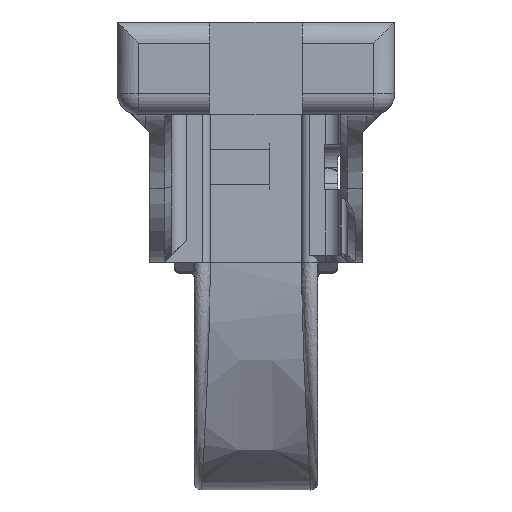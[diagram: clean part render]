
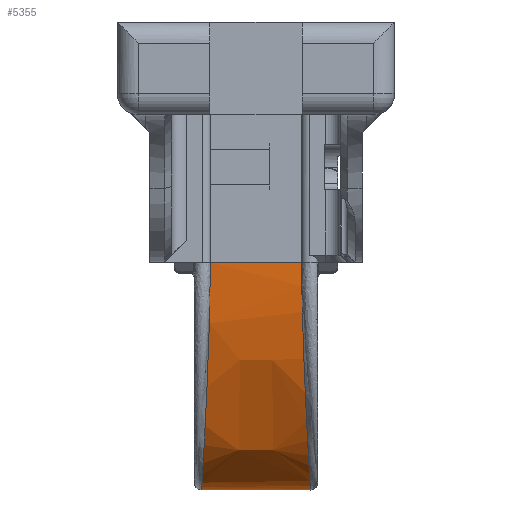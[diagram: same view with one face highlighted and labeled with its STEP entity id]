
A CAD part, left-side view. The second image highlights one B-rep face of the part: STEP entity #5355.
In plain terms, the highlighted free-form (B-spline) face has degree [3, 3] with [4, 4] control points.
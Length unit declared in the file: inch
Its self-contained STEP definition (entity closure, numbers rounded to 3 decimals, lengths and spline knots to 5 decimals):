
#70 = VERTEX_POINT ( 'NONE', #4380 ) ;
#248 = CARTESIAN_POINT ( 'NONE',  ( -0.38772, -0.25252, -3.07902 ) ) ;
#508 = CARTESIAN_POINT ( 'NONE',  ( -0.16815, -0.30113, -3.85823 ) ) ;
#726 = EDGE_CURVE ( 'NONE', #10322, #70, #4821, .T. ) ;
#775 = B_SPLINE_SURFACE_WITH_KNOTS ( 'NONE', 3, 3, ( 
 ( #8482, #3906, #8348, #7526 ),
 ( #4194, #6306, #5757, #4771 ),
 ( #4387, #3349, #3113, #1288 ),
 ( #785, #508, #248, #13104 ) ),
 .UNSPECIFIED., .F., .F., .F.,
 ( 4, 4 ),
 ( 4, 4 ),
 ( 0., 1. ),
 ( 0., 1. ),
 .UNSPECIFIED. ) ;
#785 = CARTESIAN_POINT ( 'NONE',  ( 0.31264, -0.30113, -3.85823 ) ) ;
#1165 = CARTESIAN_POINT ( 'NONE',  ( -0.38772, 0.25252, -2.59823 ) ) ;
#1271 = EDGE_LOOP ( 'NONE', ( #6556, #1324, #7472, #7667 ) ) ;
#1288 = CARTESIAN_POINT ( 'NONE',  ( -0.38772, -0.08417, -2.59823 ) ) ;
#1324 = ORIENTED_EDGE ( 'NONE', *, *, #9074, .T. ) ;
#1692 = B_SPLINE_CURVE_WITH_KNOTS ( 'NONE', 3,
 ( #6113, #6970, #6073, #6039 ),
 .UNSPECIFIED., .F., .F.,
 ( 4, 4 ),
 ( 0., 1. ),
 .UNSPECIFIED. ) ;
#1885 = CARTESIAN_POINT ( 'NONE',  ( 0.31264, 0.73097, -3.85823 ) ) ;
#2509 = CARTESIAN_POINT ( 'NONE',  ( -0.38772, -0.25252, -2.59823 ) ) ;
#2589 = DIRECTION ( 'NONE',  ( 0., 1., 0. ) ) ;
#2643 = CARTESIAN_POINT ( 'NONE',  ( -0.38772, 0., -2.59823 ) ) ;
#2877 = VERTEX_POINT ( 'NONE', #2509 ) ;
#3113 = CARTESIAN_POINT ( 'NONE',  ( -0.38772, -0.08417, -3.07902 ) ) ;
#3349 = CARTESIAN_POINT ( 'NONE',  ( -0.16815, -0.10038, -3.85823 ) ) ;
#3477 = CARTESIAN_POINT ( 'NONE',  ( -0.38772, 0.25252, -2.59823 ) ) ;
#3906 = CARTESIAN_POINT ( 'NONE',  ( -0.16815, 0.30113, -3.85823 ) ) ;
#4194 = CARTESIAN_POINT ( 'NONE',  ( 0.31264, 0.10038, -3.85823 ) ) ;
#4315 = CARTESIAN_POINT ( 'NONE',  ( 0.31264, 0.30113, -3.85823 ) ) ;
#4380 = CARTESIAN_POINT ( 'NONE',  ( 0.31264, -0.30113, -3.85823 ) ) ;
#4387 = CARTESIAN_POINT ( 'NONE',  ( 0.31264, -0.10038, -3.85823 ) ) ;
#4621 = VECTOR ( 'NONE', #12968, 39.37008 ) ;
#4771 = CARTESIAN_POINT ( 'NONE',  ( -0.38772, 0.08417, -2.59823 ) ) ;
#4796 = B_SPLINE_CURVE_WITH_KNOTS ( 'NONE', 3,
 ( #3477, #11599, #5252, #5219 ),
 .UNSPECIFIED., .F., .F.,
 ( 4, 4 ),
 ( 0., 1. ),
 .UNSPECIFIED. ) ;
#4821 = LINE ( 'NONE', #1885, #4621 ) ;
#5219 = CARTESIAN_POINT ( 'NONE',  ( 0.31264, 0.30113, -3.85823 ) ) ;
#5252 = CARTESIAN_POINT ( 'NONE',  ( -0.16815, 0.30113, -3.85823 ) ) ;
#5355 = ADVANCED_FACE ( 'NONE', ( #12349 ), #775, .T. ) ;
#5757 = CARTESIAN_POINT ( 'NONE',  ( -0.38772, 0.08417, -3.07902 ) ) ;
#6039 = CARTESIAN_POINT ( 'NONE',  ( -0.38772, -0.25252, -2.59823 ) ) ;
#6073 = CARTESIAN_POINT ( 'NONE',  ( -0.38772, -0.25252, -3.07902 ) ) ;
#6113 = CARTESIAN_POINT ( 'NONE',  ( 0.31264, -0.30113, -3.85823 ) ) ;
#6306 = CARTESIAN_POINT ( 'NONE',  ( -0.16815, 0.10038, -3.85823 ) ) ;
#6556 = ORIENTED_EDGE ( 'NONE', *, *, #726, .T. ) ;
#6875 = VERTEX_POINT ( 'NONE', #1165 ) ;
#6970 = CARTESIAN_POINT ( 'NONE',  ( -0.16815, -0.30113, -3.85823 ) ) ;
#7105 = EDGE_CURVE ( 'NONE', #6875, #10322, #4796, .T. ) ;
#7472 = ORIENTED_EDGE ( 'NONE', *, *, #8386, .T. ) ;
#7526 = CARTESIAN_POINT ( 'NONE',  ( -0.38772, 0.25252, -2.59823 ) ) ;
#7667 = ORIENTED_EDGE ( 'NONE', *, *, #7105, .T. ) ;
#8348 = CARTESIAN_POINT ( 'NONE',  ( -0.38772, 0.25252, -3.07902 ) ) ;
#8386 = EDGE_CURVE ( 'NONE', #2877, #6875, #11644, .T. ) ;
#8482 = CARTESIAN_POINT ( 'NONE',  ( 0.31264, 0.30113, -3.85823 ) ) ;
#9074 = EDGE_CURVE ( 'NONE', #70, #2877, #1692, .T. ) ;
#10322 = VERTEX_POINT ( 'NONE', #4315 ) ;
#11599 = CARTESIAN_POINT ( 'NONE',  ( -0.38772, 0.25252, -3.07902 ) ) ;
#11644 = LINE ( 'NONE', #2643, #12313 ) ;
#12313 = VECTOR ( 'NONE', #2589, 39.37008 ) ;
#12349 = FACE_OUTER_BOUND ( 'NONE', #1271, .T. ) ;
#12968 = DIRECTION ( 'NONE',  ( 0., -1., 0. ) ) ;
#13104 = CARTESIAN_POINT ( 'NONE',  ( -0.38772, -0.25252, -2.59823 ) ) ;
